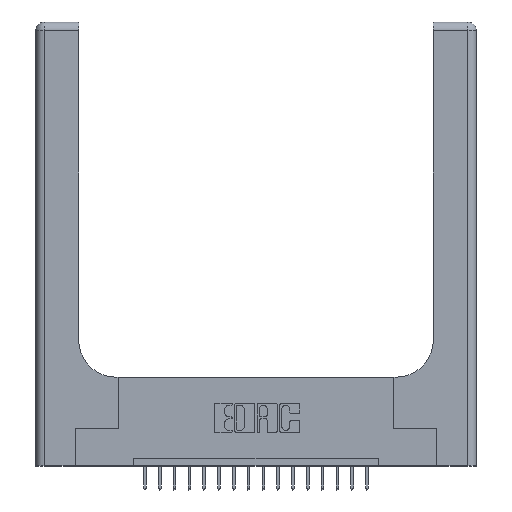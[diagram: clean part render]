
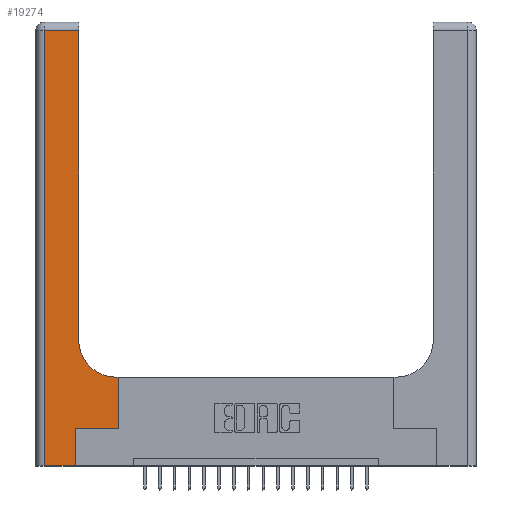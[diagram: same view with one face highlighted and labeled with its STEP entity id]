
A CAD part, top view. The second image highlights one B-rep face of the part: STEP entity #19274.
In plain terms, the highlighted planar face has unit normal (0, 0, 1).
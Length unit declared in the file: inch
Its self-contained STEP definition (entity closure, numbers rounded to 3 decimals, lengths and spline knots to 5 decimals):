
#121 = CARTESIAN_POINT ( 'NONE',  ( 0.06, 2.94, 0.37 ) ) ;
#168 = CARTESIAN_POINT ( 'NONE',  ( 0.269, 0., 0.37 ) ) ;
#225 = LINE ( 'NONE', #1243, #9022 ) ;
#298 = DIRECTION ( 'NONE',  ( -1., 0., 0. ) ) ;
#330 = DIRECTION ( 'NONE',  ( 0., -1., 0. ) ) ;
#981 = DIRECTION ( 'NONE',  ( 0., 0., -1. ) ) ;
#1219 = DIRECTION ( 'NONE',  ( 0., 1., 0. ) ) ;
#1243 = CARTESIAN_POINT ( 'NONE',  ( 0., 0., 0.37 ) ) ;
#2768 = DIRECTION ( 'NONE',  ( -1., 0., 0. ) ) ;
#2839 = CARTESIAN_POINT ( 'NONE',  ( 0., 3., 0.37 ) ) ;
#3115 = FACE_OUTER_BOUND ( 'NONE', #12592, .T. ) ;
#3641 = DIRECTION ( 'NONE',  ( -1., 0., 0. ) ) ;
#3694 = ORIENTED_EDGE ( 'NONE', *, *, #3829, .T. ) ;
#3829 = EDGE_CURVE ( 'NONE', #7349, #16386, #225, .T. ) ;
#4131 = CARTESIAN_POINT ( 'NONE',  ( 0.269, 0., 0.37 ) ) ;
#4626 = VECTOR ( 'NONE', #4924, 39.37008 ) ;
#4677 = DIRECTION ( 'NONE',  ( 1., 0., 0. ) ) ;
#4924 = DIRECTION ( 'NONE',  ( 0., 1., 0. ) ) ;
#5548 = CIRCLE ( 'NONE', #12117, 0.25 ) ;
#5835 = CARTESIAN_POINT ( 'NONE',  ( 0., 2.94, 0.37 ) ) ;
#5927 = LINE ( 'NONE', #9266, #13910 ) ;
#6245 = EDGE_CURVE ( 'NONE', #11143, #13371, #5927, .T. ) ;
#6250 = DIRECTION ( 'NONE',  ( 0., 1., 0. ) ) ;
#6555 = LINE ( 'NONE', #10621, #14551 ) ;
#6558 = CARTESIAN_POINT ( 'NONE',  ( 0.06, 3., 0.37 ) ) ;
#6908 = VECTOR ( 'NONE', #8959, 39.37008 ) ;
#7343 = ORIENTED_EDGE ( 'NONE', *, *, #9488, .T. ) ;
#7349 = VERTEX_POINT ( 'NONE', #17277 ) ;
#7679 = CARTESIAN_POINT ( 'NONE',  ( 0.2915, 0.85, 0.37 ) ) ;
#7856 = ORIENTED_EDGE ( 'NONE', *, *, #11929, .T. ) ;
#8959 = DIRECTION ( 'NONE',  ( 1., 0., 0. ) ) ;
#9022 = VECTOR ( 'NONE', #11303, 39.37008 ) ;
#9266 = CARTESIAN_POINT ( 'NONE',  ( 0.2915, 3., 0.37 ) ) ;
#9488 = EDGE_CURVE ( 'NONE', #10337, #17351, #6555, .T. ) ;
#9527 = ORIENTED_EDGE ( 'NONE', *, *, #19335, .T. ) ;
#9804 = CARTESIAN_POINT ( 'NONE',  ( 0.5415, 0.85, 0.37 ) ) ;
#10108 = VERTEX_POINT ( 'NONE', #19882 ) ;
#10332 = VECTOR ( 'NONE', #298, 39.37008 ) ;
#10337 = VERTEX_POINT ( 'NONE', #15561 ) ;
#10403 = VERTEX_POINT ( 'NONE', #121 ) ;
#10621 = CARTESIAN_POINT ( 'NONE',  ( 0.5585, 0.25, 0.37 ) ) ;
#11143 = VERTEX_POINT ( 'NONE', #7679 ) ;
#11303 = DIRECTION ( 'NONE',  ( 1., 0., 0. ) ) ;
#11699 = CARTESIAN_POINT ( 'NONE',  ( 0.5415, 0.6, 0.37 ) ) ;
#11929 = EDGE_CURVE ( 'NONE', #10403, #7349, #16186, .T. ) ;
#12117 = AXIS2_PLACEMENT_3D ( 'NONE', #9804, #12659, #4677 ) ;
#12409 = ORIENTED_EDGE ( 'NONE', *, *, #12848, .T. ) ;
#12592 = EDGE_LOOP ( 'NONE', ( #17187, #13196, #7856, #3694, #17901, #9527, #7343, #12409, #16373 ) ) ;
#12659 = DIRECTION ( 'NONE',  ( 0., 0., -1. ) ) ;
#12848 = EDGE_CURVE ( 'NONE', #17351, #13448, #15890, .T. ) ;
#13173 = VECTOR ( 'NONE', #330, 39.37008 ) ;
#13196 = ORIENTED_EDGE ( 'NONE', *, *, #14365, .T. ) ;
#13371 = VERTEX_POINT ( 'NONE', #14517 ) ;
#13448 = VERTEX_POINT ( 'NONE', #11699 ) ;
#13872 = VECTOR ( 'NONE', #3641, 39.37008 ) ;
#13910 = VECTOR ( 'NONE', #6250, 39.37008 ) ;
#14365 = EDGE_CURVE ( 'NONE', #13371, #10403, #14824, .T. ) ;
#14517 = CARTESIAN_POINT ( 'NONE',  ( 0.2915, 2.94, 0.37 ) ) ;
#14551 = VECTOR ( 'NONE', #1219, 39.37008 ) ;
#14739 = EDGE_CURVE ( 'NONE', #13448, #11143, #5548, .T. ) ;
#14742 = CARTESIAN_POINT ( 'NONE',  ( 0.5585, 0.6, 0.37 ) ) ;
#14824 = LINE ( 'NONE', #5835, #10332 ) ;
#15561 = CARTESIAN_POINT ( 'NONE',  ( 0.5585, 0.25, 0.37 ) ) ;
#15656 = PLANE ( 'NONE',  #17989 ) ;
#15890 = LINE ( 'NONE', #17956, #13872 ) ;
#16186 = LINE ( 'NONE', #6558, #13173 ) ;
#16373 = ORIENTED_EDGE ( 'NONE', *, *, #14739, .T. ) ;
#16386 = VERTEX_POINT ( 'NONE', #4131 ) ;
#16403 = LINE ( 'NONE', #17062, #6908 ) ;
#16687 = LINE ( 'NONE', #168, #4626 ) ;
#17062 = CARTESIAN_POINT ( 'NONE',  ( 0.269, 0.25, 0.37 ) ) ;
#17187 = ORIENTED_EDGE ( 'NONE', *, *, #6245, .T. ) ;
#17277 = CARTESIAN_POINT ( 'NONE',  ( 0.06, 0., 0.37 ) ) ;
#17351 = VERTEX_POINT ( 'NONE', #14742 ) ;
#17901 = ORIENTED_EDGE ( 'NONE', *, *, #18955, .T. ) ;
#17956 = CARTESIAN_POINT ( 'NONE',  ( 0.2915, 0.6, 0.37 ) ) ;
#17989 = AXIS2_PLACEMENT_3D ( 'NONE', #2839, #981, #2768 ) ;
#18955 = EDGE_CURVE ( 'NONE', #16386, #10108, #16687, .T. ) ;
#19274 = ADVANCED_FACE ( 'NONE', ( #3115 ), #15656, .F. ) ;
#19335 = EDGE_CURVE ( 'NONE', #10108, #10337, #16403, .T. ) ;
#19882 = CARTESIAN_POINT ( 'NONE',  ( 0.269, 0.25, 0.37 ) ) ;
